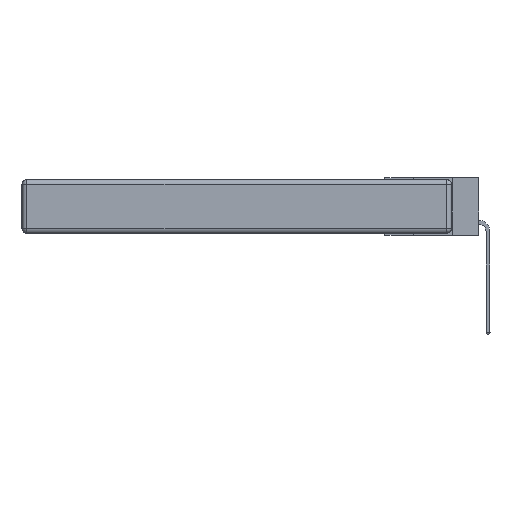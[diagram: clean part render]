
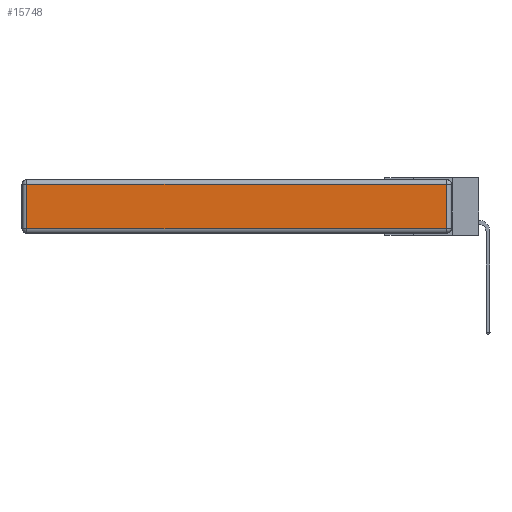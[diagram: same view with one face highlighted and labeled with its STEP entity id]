
A CAD part, left-side view. The second image highlights one B-rep face of the part: STEP entity #15748.
In plain terms, the highlighted planar face has unit normal (-1, 0, 0).
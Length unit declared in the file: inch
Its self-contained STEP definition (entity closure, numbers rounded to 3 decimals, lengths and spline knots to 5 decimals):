
#1483 = CARTESIAN_POINT ( 'NONE',  ( 0., 2.75, -0.03 ) ) ;
#1832 = ORIENTED_EDGE ( 'NONE', *, *, #14851, .T. ) ;
#2214 = PLANE ( 'NONE',  #8447 ) ;
#3239 = CARTESIAN_POINT ( 'NONE',  ( 0., 0.03, -0.343 ) ) ;
#3529 = CARTESIAN_POINT ( 'NONE',  ( 0., 2.72, -0.343 ) ) ;
#3582 = CARTESIAN_POINT ( 'NONE',  ( 0., 2.72, -0.03 ) ) ;
#4459 = VERTEX_POINT ( 'NONE', #3582 ) ;
#4708 = DIRECTION ( 'NONE',  ( 0., 0., 1. ) ) ;
#4943 = EDGE_CURVE ( 'NONE', #11286, #18213, #17668, .T. ) ;
#5824 = LINE ( 'NONE', #16101, #18563 ) ;
#6259 = CARTESIAN_POINT ( 'NONE',  ( 0., 2.72, -0.313 ) ) ;
#6291 = ORIENTED_EDGE ( 'NONE', *, *, #9905, .T. ) ;
#6762 = LINE ( 'NONE', #3529, #16312 ) ;
#7376 = DIRECTION ( 'NONE',  ( 0., -1., 0. ) ) ;
#8012 = CARTESIAN_POINT ( 'NONE',  ( 0., 0.03, -0.313 ) ) ;
#8447 = AXIS2_PLACEMENT_3D ( 'NONE', #11125, #16969, #13864 ) ;
#8459 = DIRECTION ( 'NONE',  ( 0., 1., 0. ) ) ;
#8882 = VECTOR ( 'NONE', #8459, 39.37008 ) ;
#9905 = EDGE_CURVE ( 'NONE', #4459, #11785, #6762, .T. ) ;
#10021 = FACE_OUTER_BOUND ( 'NONE', #16737, .T. ) ;
#10389 = EDGE_CURVE ( 'NONE', #11785, #11286, #5824, .T. ) ;
#11086 = ORIENTED_EDGE ( 'NONE', *, *, #4943, .T. ) ;
#11125 = CARTESIAN_POINT ( 'NONE',  ( 0., 0., -0.343 ) ) ;
#11286 = VERTEX_POINT ( 'NONE', #8012 ) ;
#11785 = VERTEX_POINT ( 'NONE', #6259 ) ;
#12593 = ORIENTED_EDGE ( 'NONE', *, *, #10389, .T. ) ;
#13681 = DIRECTION ( 'NONE',  ( 0., 0., -1. ) ) ;
#13864 = DIRECTION ( 'NONE',  ( 0., 0., 1. ) ) ;
#14851 = EDGE_CURVE ( 'NONE', #18213, #4459, #16413, .T. ) ;
#15164 = VECTOR ( 'NONE', #4708, 39.37008 ) ;
#15748 = ADVANCED_FACE ( 'NONE', ( #10021 ), #2214, .T. ) ;
#16057 = CARTESIAN_POINT ( 'NONE',  ( 0., 0.03, -0.03 ) ) ;
#16101 = CARTESIAN_POINT ( 'NONE',  ( 0., 0., -0.313 ) ) ;
#16312 = VECTOR ( 'NONE', #13681, 39.37008 ) ;
#16413 = LINE ( 'NONE', #1483, #8882 ) ;
#16737 = EDGE_LOOP ( 'NONE', ( #12593, #11086, #1832, #6291 ) ) ;
#16969 = DIRECTION ( 'NONE',  ( -1., 0., 0. ) ) ;
#17668 = LINE ( 'NONE', #3239, #15164 ) ;
#18213 = VERTEX_POINT ( 'NONE', #16057 ) ;
#18563 = VECTOR ( 'NONE', #7376, 39.37008 ) ;
